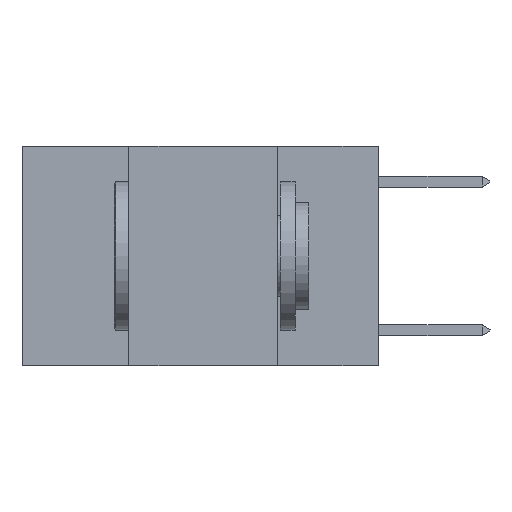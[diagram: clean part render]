
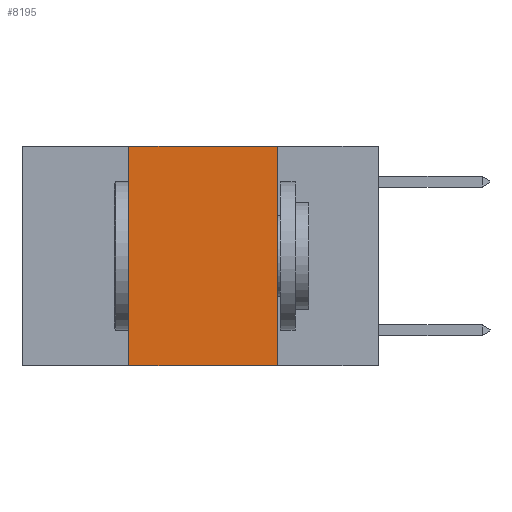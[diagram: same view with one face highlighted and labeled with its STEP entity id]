
A CAD part, left-side view. The second image highlights one B-rep face of the part: STEP entity #8195.
In plain terms, the highlighted planar face has unit normal (-1, 0, 0).
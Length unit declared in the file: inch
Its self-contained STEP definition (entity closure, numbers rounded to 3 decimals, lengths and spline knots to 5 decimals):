
#229 = ORIENTED_EDGE ( 'NONE', *, *, #20466, .F. ) ;
#251 = ORIENTED_EDGE ( 'NONE', *, *, #5708, .T. ) ;
#431 = DIRECTION ( 'NONE',  ( 0., -1., 0. ) ) ;
#3980 = DIRECTION ( 'NONE',  ( 0., 0., -1. ) ) ;
#4194 = DIRECTION ( 'NONE',  ( 1., 0., 0. ) ) ;
#4553 = EDGE_LOOP ( 'NONE', ( #26181, #29291, #229, #251 ) ) ;
#5347 = DIRECTION ( 'NONE',  ( 0., -1., 0. ) ) ;
#5708 = EDGE_CURVE ( 'NONE', #9000, #16594, #29258, .T. ) ;
#6679 = VECTOR ( 'NONE', #8267, 39.37008 ) ;
#6902 = FACE_OUTER_BOUND ( 'NONE', #4553, .T. ) ;
#8195 = ADVANCED_FACE ( 'NONE', ( #6902 ), #20523, .F. ) ;
#8267 = DIRECTION ( 'NONE',  ( 0., 0., 1. ) ) ;
#9000 = VERTEX_POINT ( 'NONE', #9188 ) ;
#9188 = CARTESIAN_POINT ( 'NONE',  ( 0., 0.42, -0.37 ) ) ;
#11674 = LINE ( 'NONE', #12097, #29295 ) ;
#12097 = CARTESIAN_POINT ( 'NONE',  ( 0., 0.6, 0. ) ) ;
#13037 = CARTESIAN_POINT ( 'NONE',  ( 0., 0.17, -0.37 ) ) ;
#14972 = LINE ( 'NONE', #27183, #19741 ) ;
#16594 = VERTEX_POINT ( 'NONE', #13037 ) ;
#17888 = VERTEX_POINT ( 'NONE', #29120 ) ;
#19741 = VECTOR ( 'NONE', #3980, 39.37008 ) ;
#20072 = AXIS2_PLACEMENT_3D ( 'NONE', #27369, #4194, #20624 ) ;
#20466 = EDGE_CURVE ( 'NONE', #9000, #20825, #29773, .T. ) ;
#20523 = PLANE ( 'NONE',  #20072 ) ;
#20624 = DIRECTION ( 'NONE',  ( 0., 0., -1. ) ) ;
#20825 = VERTEX_POINT ( 'NONE', #28364 ) ;
#24598 = CARTESIAN_POINT ( 'NONE',  ( 0., 0.42, 0. ) ) ;
#25069 = EDGE_CURVE ( 'NONE', #17888, #16594, #14972, .T. ) ;
#25375 = EDGE_CURVE ( 'NONE', #20825, #17888, #11674, .T. ) ;
#26181 = ORIENTED_EDGE ( 'NONE', *, *, #25069, .F. ) ;
#27183 = CARTESIAN_POINT ( 'NONE',  ( 0., 0.17, 0. ) ) ;
#27369 = CARTESIAN_POINT ( 'NONE',  ( 0., 0.6, 0. ) ) ;
#28364 = CARTESIAN_POINT ( 'NONE',  ( 0., 0.42, 0. ) ) ;
#28440 = CARTESIAN_POINT ( 'NONE',  ( 0., 0.6, -0.37 ) ) ;
#29062 = VECTOR ( 'NONE', #5347, 39.37008 ) ;
#29120 = CARTESIAN_POINT ( 'NONE',  ( 0., 0.17, 0. ) ) ;
#29258 = LINE ( 'NONE', #28440, #29062 ) ;
#29291 = ORIENTED_EDGE ( 'NONE', *, *, #25375, .F. ) ;
#29295 = VECTOR ( 'NONE', #431, 39.37008 ) ;
#29773 = LINE ( 'NONE', #24598, #6679 ) ;
